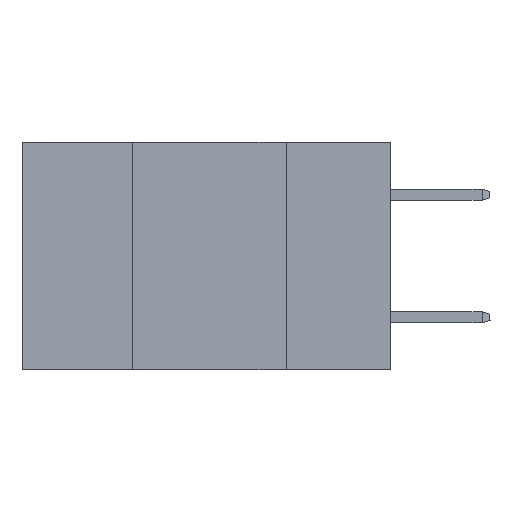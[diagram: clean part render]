
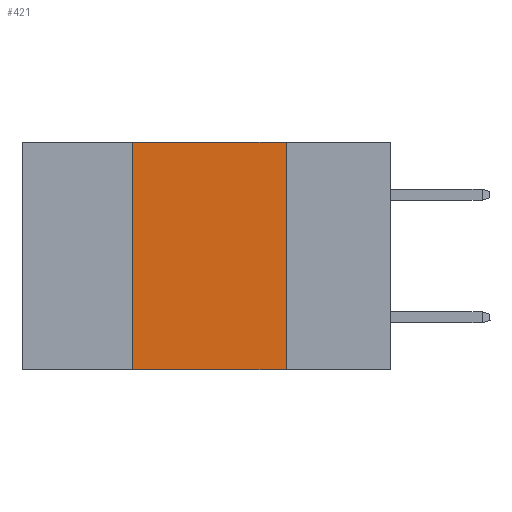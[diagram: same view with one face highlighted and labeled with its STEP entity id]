
A CAD part, left-side view. The second image highlights one B-rep face of the part: STEP entity #421.
In plain terms, the highlighted planar face has unit normal (-1, 0, 0).
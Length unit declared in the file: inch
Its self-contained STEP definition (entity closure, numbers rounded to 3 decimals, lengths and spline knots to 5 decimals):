
#116 = VERTEX_POINT ( 'NONE', #133 ) ;
#133 = CARTESIAN_POINT ( 'NONE',  ( 0., 0.17, -0.37 ) ) ;
#421 = ADVANCED_FACE ( 'NONE', ( #9423 ), #9080, .F. ) ;
#583 = ORIENTED_EDGE ( 'NONE', *, *, #9528, .F. ) ;
#1511 = LINE ( 'NONE', #2244, #10746 ) ;
#1520 = EDGE_CURVE ( 'NONE', #4452, #116, #1511, .T. ) ;
#1934 = EDGE_CURVE ( 'NONE', #4452, #9196, #5967, .T. ) ;
#2154 = DIRECTION ( 'NONE',  ( 0., 0., -1. ) ) ;
#2244 = CARTESIAN_POINT ( 'NONE',  ( 0., 0.6, -0.37 ) ) ;
#2591 = CARTESIAN_POINT ( 'NONE',  ( 0., 0.42, -0.37 ) ) ;
#2806 = LINE ( 'NONE', #8139, #7092 ) ;
#3028 = EDGE_LOOP ( 'NONE', ( #583, #7625, #5688, #7892 ) ) ;
#3459 = CARTESIAN_POINT ( 'NONE',  ( 0., 0.42, 0. ) ) ;
#3908 = CARTESIAN_POINT ( 'NONE',  ( 0., 0.6, 0. ) ) ;
#3964 = VERTEX_POINT ( 'NONE', #10987 ) ;
#4168 = DIRECTION ( 'NONE',  ( 0., -1., 0. ) ) ;
#4215 = DIRECTION ( 'NONE',  ( 0., -1., 0. ) ) ;
#4452 = VERTEX_POINT ( 'NONE', #2591 ) ;
#4758 = DIRECTION ( 'NONE',  ( 1., 0., 0. ) ) ;
#5688 = ORIENTED_EDGE ( 'NONE', *, *, #1934, .F. ) ;
#5967 = LINE ( 'NONE', #10371, #10246 ) ;
#6390 = EDGE_CURVE ( 'NONE', #9196, #3964, #10008, .T. ) ;
#7092 = VECTOR ( 'NONE', #2154, 39.37008 ) ;
#7625 = ORIENTED_EDGE ( 'NONE', *, *, #6390, .F. ) ;
#7892 = ORIENTED_EDGE ( 'NONE', *, *, #1520, .T. ) ;
#8139 = CARTESIAN_POINT ( 'NONE',  ( 0., 0.17, 0. ) ) ;
#8371 = CARTESIAN_POINT ( 'NONE',  ( 0., 0.6, 0. ) ) ;
#9080 = PLANE ( 'NONE',  #10617 ) ;
#9196 = VERTEX_POINT ( 'NONE', #3459 ) ;
#9423 = FACE_OUTER_BOUND ( 'NONE', #3028, .T. ) ;
#9528 = EDGE_CURVE ( 'NONE', #3964, #116, #2806, .T. ) ;
#9750 = VECTOR ( 'NONE', #4168, 39.37008 ) ;
#10008 = LINE ( 'NONE', #8371, #9750 ) ;
#10246 = VECTOR ( 'NONE', #10384, 39.37008 ) ;
#10338 = DIRECTION ( 'NONE',  ( 0., 0., -1. ) ) ;
#10371 = CARTESIAN_POINT ( 'NONE',  ( 0., 0.42, 0. ) ) ;
#10384 = DIRECTION ( 'NONE',  ( 0., 0., 1. ) ) ;
#10617 = AXIS2_PLACEMENT_3D ( 'NONE', #3908, #4758, #10338 ) ;
#10746 = VECTOR ( 'NONE', #4215, 39.37008 ) ;
#10987 = CARTESIAN_POINT ( 'NONE',  ( 0., 0.17, 0. ) ) ;
